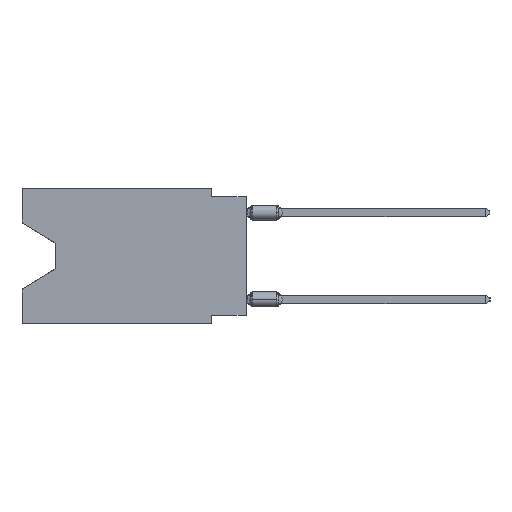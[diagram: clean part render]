
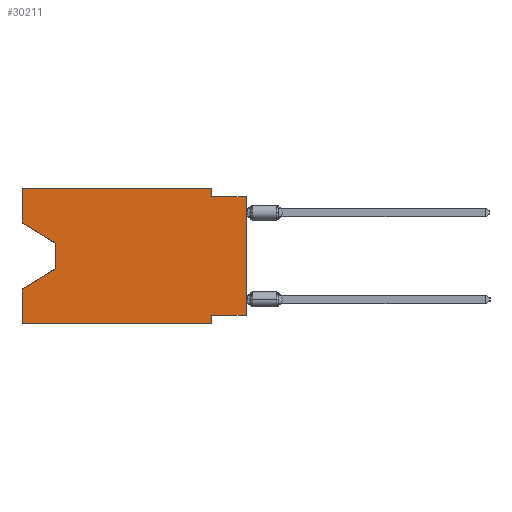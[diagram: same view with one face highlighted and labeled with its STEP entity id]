
A CAD part, left-side view. The second image highlights one B-rep face of the part: STEP entity #30211.
In plain terms, the highlighted planar face has unit normal (-1, 0, 0).
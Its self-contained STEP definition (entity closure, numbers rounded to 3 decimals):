
#101 = CARTESIAN_POINT ( 'NONE',  ( 0., 16.383, -7.36 ) ) ;
#639 = EDGE_CURVE ( 'NONE', #21786, #31515, #6001, .T. ) ;
#1191 = ORIENTED_EDGE ( 'NONE', *, *, #36185, .F. ) ;
#1612 = CARTESIAN_POINT ( 'NONE',  ( 0., 16.383, -9.906 ) ) ;
#1846 = LINE ( 'NONE', #23773, #4326 ) ;
#2678 = DIRECTION ( 'NONE',  ( 1., 0., 0. ) ) ;
#3344 = LINE ( 'NONE', #17711, #45341 ) ;
#4326 = VECTOR ( 'NONE', #12697, 1000. ) ;
#4569 = LINE ( 'NONE', #44429, #36407 ) ;
#4708 = LINE ( 'NONE', #19066, #37728 ) ;
#5267 = AXIS2_PLACEMENT_3D ( 'NONE', #22969, #2678, #31455 ) ;
#5434 = CARTESIAN_POINT ( 'NONE',  ( 0., 0., -9.271 ) ) ;
#6001 = LINE ( 'NONE', #31233, #36472 ) ;
#6221 = ORIENTED_EDGE ( 'NONE', *, *, #41225, .F. ) ;
#6229 = VERTEX_POINT ( 'NONE', #41178 ) ;
#7346 = VERTEX_POINT ( 'NONE', #28791 ) ;
#7433 = VECTOR ( 'NONE', #27444, 1000. ) ;
#7937 = EDGE_CURVE ( 'NONE', #20030, #21162, #30993, .T. ) ;
#8505 = EDGE_LOOP ( 'NONE', ( #16947, #46258, #26997, #1191, #16999, #11910, #17623, #10887, #34532, #24822, #26066, #6221 ) ) ;
#8604 = PLANE ( 'NONE',  #5267 ) ;
#9708 = DIRECTION ( 'NONE',  ( 0., 0., -1. ) ) ;
#10887 = ORIENTED_EDGE ( 'NONE', *, *, #21661, .T. ) ;
#11910 = ORIENTED_EDGE ( 'NONE', *, *, #639, .F. ) ;
#12697 = DIRECTION ( 'NONE',  ( 0., 0., 1. ) ) ;
#13053 = CARTESIAN_POINT ( 'NONE',  ( 0., 13.97, -5.893 ) ) ;
#14822 = DIRECTION ( 'NONE',  ( 0., -0.855, -0.519 ) ) ;
#14911 = CARTESIAN_POINT ( 'NONE',  ( 0., 2.54, -0.635 ) ) ;
#14962 = EDGE_CURVE ( 'NONE', #31273, #40983, #4708, .T. ) ;
#15309 = VECTOR ( 'NONE', #19521, 1000. ) ;
#16450 = CARTESIAN_POINT ( 'NONE',  ( 0., 0., -0.635 ) ) ;
#16528 = LINE ( 'NONE', #42003, #37323 ) ;
#16947 = ORIENTED_EDGE ( 'NONE', *, *, #19047, .T. ) ;
#16999 = ORIENTED_EDGE ( 'NONE', *, *, #41684, .T. ) ;
#17138 = LINE ( 'NONE', #16450, #35469 ) ;
#17623 = ORIENTED_EDGE ( 'NONE', *, *, #43880, .F. ) ;
#17642 = CARTESIAN_POINT ( 'NONE',  ( 0., 16.383, -9.906 ) ) ;
#17711 = CARTESIAN_POINT ( 'NONE',  ( 0., 0., 0. ) ) ;
#17760 = CARTESIAN_POINT ( 'NONE',  ( 0., 13.97, -5.893 ) ) ;
#19047 = EDGE_CURVE ( 'NONE', #46323, #7346, #44301, .T. ) ;
#19066 = CARTESIAN_POINT ( 'NONE',  ( 0., 2.54, 0. ) ) ;
#19521 = DIRECTION ( 'NONE',  ( 0., -1., 0. ) ) ;
#20030 = VERTEX_POINT ( 'NONE', #17760 ) ;
#20958 = DIRECTION ( 'NONE',  ( 0., -1., 0. ) ) ;
#21162 = VERTEX_POINT ( 'NONE', #101 ) ;
#21661 = EDGE_CURVE ( 'NONE', #38387, #30803, #3344, .T. ) ;
#21786 = VERTEX_POINT ( 'NONE', #37286 ) ;
#22154 = EDGE_CURVE ( 'NONE', #6229, #31273, #29704, .T. ) ;
#22489 = DIRECTION ( 'NONE',  ( 0., 1., 0. ) ) ;
#22844 = DIRECTION ( 'NONE',  ( 0., 0., -1. ) ) ;
#22969 = CARTESIAN_POINT ( 'NONE',  ( 0., 16.383, 0. ) ) ;
#23773 = CARTESIAN_POINT ( 'NONE',  ( 0., 16.383, 0. ) ) ;
#23779 = VECTOR ( 'NONE', #14822, 1000. ) ;
#24001 = DIRECTION ( 'NONE',  ( 0., 0., 1. ) ) ;
#24822 = ORIENTED_EDGE ( 'NONE', *, *, #14962, .F. ) ;
#24927 = EDGE_CURVE ( 'NONE', #7346, #20030, #16528, .T. ) ;
#25203 = CARTESIAN_POINT ( 'NONE',  ( 0., 16.383, -2.546 ) ) ;
#26066 = ORIENTED_EDGE ( 'NONE', *, *, #22154, .F. ) ;
#26997 = ORIENTED_EDGE ( 'NONE', *, *, #7937, .T. ) ;
#27444 = DIRECTION ( 'NONE',  ( 0., 0.855, -0.519 ) ) ;
#27828 = VERTEX_POINT ( 'NONE', #1612 ) ;
#28452 = CARTESIAN_POINT ( 'NONE',  ( 0., 2.54, -9.906 ) ) ;
#28791 = CARTESIAN_POINT ( 'NONE',  ( 0., 13.97, -4.013 ) ) ;
#29704 = LINE ( 'NONE', #33916, #15309 ) ;
#29940 = VECTOR ( 'NONE', #20958, 1000. ) ;
#30211 = ADVANCED_FACE ( 'NONE', ( #40915 ), #8604, .F. ) ;
#30803 = VERTEX_POINT ( 'NONE', #46487 ) ;
#30993 = LINE ( 'NONE', #13053, #7433 ) ;
#31233 = CARTESIAN_POINT ( 'NONE',  ( 0., 2.54, -9.906 ) ) ;
#31273 = VERTEX_POINT ( 'NONE', #43814 ) ;
#31455 = DIRECTION ( 'NONE',  ( 0., 0., -1. ) ) ;
#31515 = VERTEX_POINT ( 'NONE', #28452 ) ;
#33916 = CARTESIAN_POINT ( 'NONE',  ( 0., 16.383, 0. ) ) ;
#34037 = CARTESIAN_POINT ( 'NONE',  ( 0., 16.383, -2.546 ) ) ;
#34532 = ORIENTED_EDGE ( 'NONE', *, *, #35008, .F. ) ;
#35008 = EDGE_CURVE ( 'NONE', #40983, #30803, #17138, .T. ) ;
#35469 = VECTOR ( 'NONE', #45452, 1000. ) ;
#36128 = DIRECTION ( 'NONE',  ( 0., 0., 1. ) ) ;
#36185 = EDGE_CURVE ( 'NONE', #27828, #21162, #38618, .T. ) ;
#36407 = VECTOR ( 'NONE', #22489, 1000. ) ;
#36472 = VECTOR ( 'NONE', #44910, 1000. ) ;
#37286 = CARTESIAN_POINT ( 'NONE',  ( 0., 2.54, -9.271 ) ) ;
#37323 = VECTOR ( 'NONE', #9708, 1000. ) ;
#37728 = VECTOR ( 'NONE', #22844, 1000. ) ;
#38387 = VERTEX_POINT ( 'NONE', #5434 ) ;
#38618 = LINE ( 'NONE', #42619, #39319 ) ;
#38888 = LINE ( 'NONE', #17642, #29940 ) ;
#39319 = VECTOR ( 'NONE', #24001, 1000. ) ;
#40915 = FACE_OUTER_BOUND ( 'NONE', #8505, .T. ) ;
#40983 = VERTEX_POINT ( 'NONE', #14911 ) ;
#41178 = CARTESIAN_POINT ( 'NONE',  ( 0., 16.383, 0. ) ) ;
#41225 = EDGE_CURVE ( 'NONE', #46323, #6229, #1846, .T. ) ;
#41684 = EDGE_CURVE ( 'NONE', #27828, #31515, #38888, .T. ) ;
#42003 = CARTESIAN_POINT ( 'NONE',  ( 0., 13.97, -4.013 ) ) ;
#42619 = CARTESIAN_POINT ( 'NONE',  ( 0., 16.383, 0. ) ) ;
#43814 = CARTESIAN_POINT ( 'NONE',  ( 0., 2.54, 0. ) ) ;
#43880 = EDGE_CURVE ( 'NONE', #38387, #21786, #4569, .T. ) ;
#44301 = LINE ( 'NONE', #25203, #23779 ) ;
#44429 = CARTESIAN_POINT ( 'NONE',  ( 0., 0., -9.271 ) ) ;
#44910 = DIRECTION ( 'NONE',  ( 0., 0., -1. ) ) ;
#45341 = VECTOR ( 'NONE', #36128, 1000. ) ;
#45452 = DIRECTION ( 'NONE',  ( 0., -1., 0. ) ) ;
#46258 = ORIENTED_EDGE ( 'NONE', *, *, #24927, .T. ) ;
#46323 = VERTEX_POINT ( 'NONE', #34037 ) ;
#46487 = CARTESIAN_POINT ( 'NONE',  ( 0., 0., -0.635 ) ) ;
